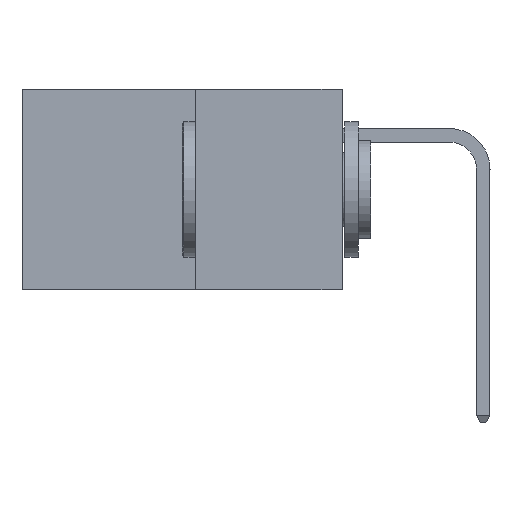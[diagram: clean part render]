
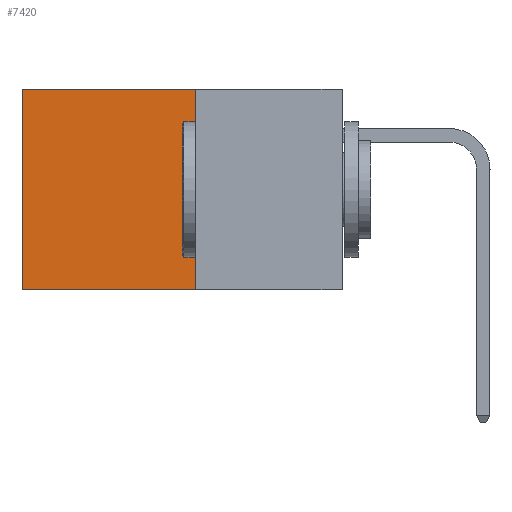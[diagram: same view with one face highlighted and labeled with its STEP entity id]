
A CAD part, left-side view. The second image highlights one B-rep face of the part: STEP entity #7420.
In plain terms, the highlighted planar face has unit normal (-1, 0, 0).
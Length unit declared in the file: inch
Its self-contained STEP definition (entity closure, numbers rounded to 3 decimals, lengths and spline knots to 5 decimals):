
#748 = DIRECTION ( 'NONE',  ( 0., 1., 0. ) ) ;
#1540 = DIRECTION ( 'NONE',  ( 0., 1., 0. ) ) ;
#1840 = VECTOR ( 'NONE', #11033, 39.37008 ) ;
#1855 = CARTESIAN_POINT ( 'NONE',  ( 0.277, 0.59, 0. ) ) ;
#3698 = CARTESIAN_POINT ( 'NONE',  ( 0.277, 0.59, -0.37 ) ) ;
#3815 = PLANE ( 'NONE',  #4080 ) ;
#4080 = AXIS2_PLACEMENT_3D ( 'NONE', #5452, #7072, #17934 ) ;
#4218 = ORIENTED_EDGE ( 'NONE', *, *, #12892, .F. ) ;
#4705 = VERTEX_POINT ( 'NONE', #7000 ) ;
#5310 = EDGE_CURVE ( 'NONE', #4705, #11384, #6184, .T. ) ;
#5321 = VECTOR ( 'NONE', #17841, 39.37008 ) ;
#5452 = CARTESIAN_POINT ( 'NONE',  ( 0.277, 0.27, -0.37 ) ) ;
#6181 = CARTESIAN_POINT ( 'NONE',  ( 0.277, 0.27, -0.37 ) ) ;
#6184 = LINE ( 'NONE', #11197, #1840 ) ;
#7000 = CARTESIAN_POINT ( 'NONE',  ( 0.277, 0.27, 0. ) ) ;
#7072 = DIRECTION ( 'NONE',  ( 1., 0., 0. ) ) ;
#7420 = ADVANCED_FACE ( 'NONE', ( #8315 ), #3815, .F. ) ;
#8315 = FACE_OUTER_BOUND ( 'NONE', #15764, .T. ) ;
#8492 = ORIENTED_EDGE ( 'NONE', *, *, #5310, .F. ) ;
#9252 = LINE ( 'NONE', #12041, #12915 ) ;
#9453 = EDGE_CURVE ( 'NONE', #4705, #10304, #9252, .T. ) ;
#9546 = LINE ( 'NONE', #3698, #5321 ) ;
#10304 = VERTEX_POINT ( 'NONE', #1855 ) ;
#10868 = VECTOR ( 'NONE', #1540, 39.37008 ) ;
#11033 = DIRECTION ( 'NONE',  ( 0., 0., -1. ) ) ;
#11197 = CARTESIAN_POINT ( 'NONE',  ( 0.277, 0.27, -0.37 ) ) ;
#11311 = CARTESIAN_POINT ( 'NONE',  ( 0.277, 0.59, -0.37 ) ) ;
#11384 = VERTEX_POINT ( 'NONE', #6181 ) ;
#11524 = VERTEX_POINT ( 'NONE', #11311 ) ;
#12041 = CARTESIAN_POINT ( 'NONE',  ( 0.277, 0.27, 0. ) ) ;
#12892 = EDGE_CURVE ( 'NONE', #11384, #11524, #15473, .T. ) ;
#12915 = VECTOR ( 'NONE', #748, 39.37008 ) ;
#15473 = LINE ( 'NONE', #17299, #10868 ) ;
#15764 = EDGE_LOOP ( 'NONE', ( #20360, #4218, #8492, #17228 ) ) ;
#16454 = EDGE_CURVE ( 'NONE', #10304, #11524, #9546, .T. ) ;
#17228 = ORIENTED_EDGE ( 'NONE', *, *, #9453, .T. ) ;
#17299 = CARTESIAN_POINT ( 'NONE',  ( 0.277, 0.27, -0.37 ) ) ;
#17841 = DIRECTION ( 'NONE',  ( 0., 0., -1. ) ) ;
#17934 = DIRECTION ( 'NONE',  ( 0., 0., -1. ) ) ;
#20360 = ORIENTED_EDGE ( 'NONE', *, *, #16454, .T. ) ;
